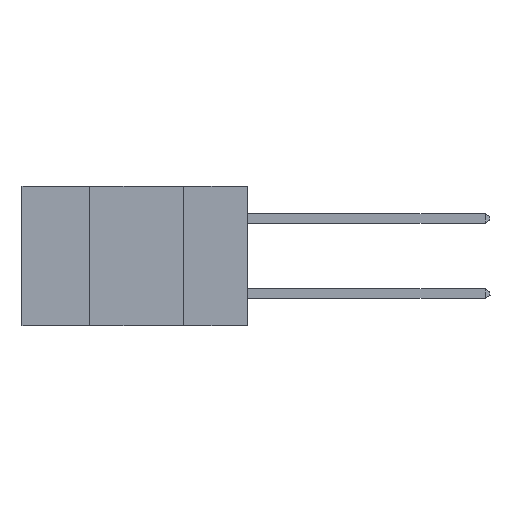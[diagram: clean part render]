
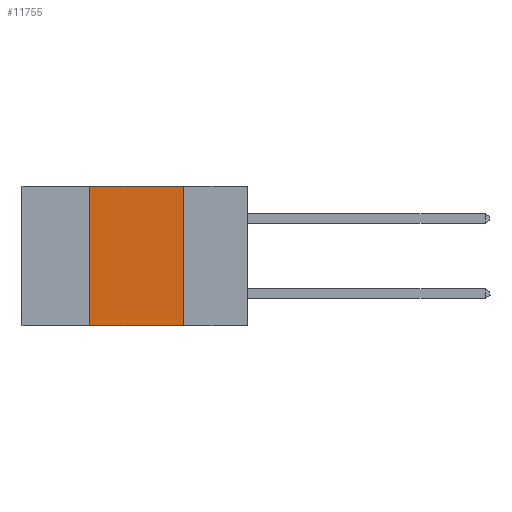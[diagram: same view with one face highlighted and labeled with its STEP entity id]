
A CAD part, left-side view. The second image highlights one B-rep face of the part: STEP entity #11755.
In plain terms, the highlighted planar face has unit normal (-1, 0, 0).
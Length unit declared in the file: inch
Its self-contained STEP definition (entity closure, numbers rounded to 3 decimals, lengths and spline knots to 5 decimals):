
#196 = VERTEX_POINT ( 'NONE', #7365 ) ;
#606 = LINE ( 'NONE', #3629, #10894 ) ;
#891 = VECTOR ( 'NONE', #5057, 39.37008 ) ;
#1324 = VERTEX_POINT ( 'NONE', #12717 ) ;
#1390 = FACE_OUTER_BOUND ( 'NONE', #9015, .T. ) ;
#1407 = DIRECTION ( 'NONE',  ( 0., 0., -1. ) ) ;
#2841 = CARTESIAN_POINT ( 'NONE',  ( 0., 0.6, -0.37 ) ) ;
#3629 = CARTESIAN_POINT ( 'NONE',  ( 0., 0.17, 0. ) ) ;
#4467 = CARTESIAN_POINT ( 'NONE',  ( 0., 0.42, 0. ) ) ;
#5057 = DIRECTION ( 'NONE',  ( 0., -1., 0. ) ) ;
#5232 = ORIENTED_EDGE ( 'NONE', *, *, #11039, .F. ) ;
#5390 = LINE ( 'NONE', #11284, #9431 ) ;
#5889 = AXIS2_PLACEMENT_3D ( 'NONE', #7102, #6124, #6033 ) ;
#6033 = DIRECTION ( 'NONE',  ( 0., 0., -1. ) ) ;
#6124 = DIRECTION ( 'NONE',  ( 1., 0., 0. ) ) ;
#6294 = EDGE_CURVE ( 'NONE', #196, #1324, #606, .T. ) ;
#6792 = EDGE_CURVE ( 'NONE', #14281, #1324, #11719, .T. ) ;
#7102 = CARTESIAN_POINT ( 'NONE',  ( 0., 0.6, 0. ) ) ;
#7365 = CARTESIAN_POINT ( 'NONE',  ( 0., 0.17, 0. ) ) ;
#9015 = EDGE_LOOP ( 'NONE', ( #10864, #5232, #11539, #10907 ) ) ;
#9245 = EDGE_CURVE ( 'NONE', #14281, #13262, #5390, .T. ) ;
#9431 = VECTOR ( 'NONE', #13831, 39.37008 ) ;
#10849 = LINE ( 'NONE', #12293, #11042 ) ;
#10864 = ORIENTED_EDGE ( 'NONE', *, *, #6294, .F. ) ;
#10894 = VECTOR ( 'NONE', #1407, 39.37008 ) ;
#10907 = ORIENTED_EDGE ( 'NONE', *, *, #6792, .T. ) ;
#11039 = EDGE_CURVE ( 'NONE', #13262, #196, #10849, .T. ) ;
#11042 = VECTOR ( 'NONE', #11052, 39.37008 ) ;
#11052 = DIRECTION ( 'NONE',  ( 0., -1., 0. ) ) ;
#11284 = CARTESIAN_POINT ( 'NONE',  ( 0., 0.42, 0. ) ) ;
#11539 = ORIENTED_EDGE ( 'NONE', *, *, #9245, .F. ) ;
#11719 = LINE ( 'NONE', #2841, #891 ) ;
#11755 = ADVANCED_FACE ( 'NONE', ( #1390 ), #12870, .F. ) ;
#12293 = CARTESIAN_POINT ( 'NONE',  ( 0., 0.6, 0. ) ) ;
#12349 = CARTESIAN_POINT ( 'NONE',  ( 0., 0.42, -0.37 ) ) ;
#12717 = CARTESIAN_POINT ( 'NONE',  ( 0., 0.17, -0.37 ) ) ;
#12870 = PLANE ( 'NONE',  #5889 ) ;
#13262 = VERTEX_POINT ( 'NONE', #4467 ) ;
#13831 = DIRECTION ( 'NONE',  ( 0., 0., 1. ) ) ;
#14281 = VERTEX_POINT ( 'NONE', #12349 ) ;
